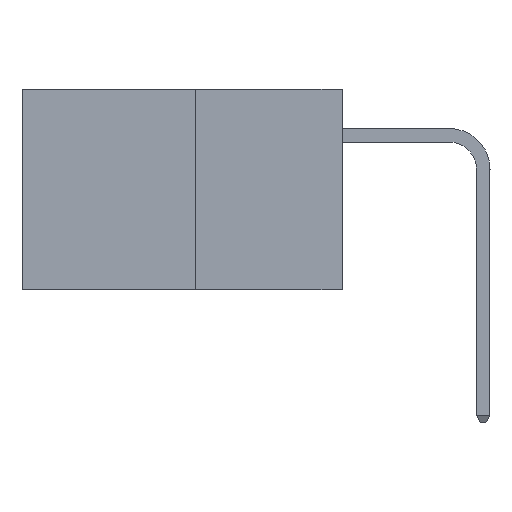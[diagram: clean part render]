
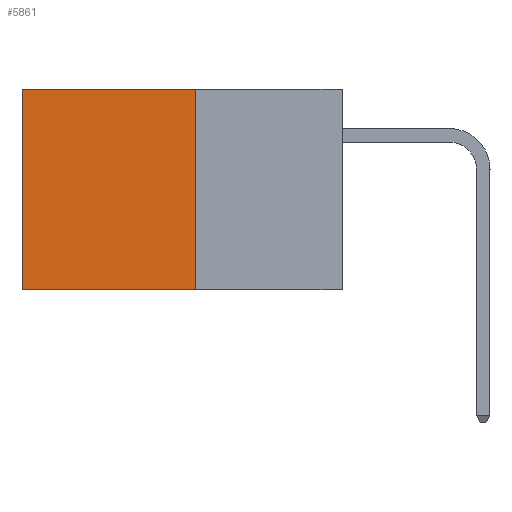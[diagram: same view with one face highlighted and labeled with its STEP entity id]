
A CAD part, left-side view. The second image highlights one B-rep face of the part: STEP entity #5861.
In plain terms, the highlighted planar face has unit normal (-1, 0, 0).
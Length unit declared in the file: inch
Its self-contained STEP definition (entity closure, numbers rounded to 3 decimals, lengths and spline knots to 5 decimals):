
#667 = VERTEX_POINT ( 'NONE', #10257 ) ;
#839 = CARTESIAN_POINT ( 'NONE',  ( 0.277, 0.27, 0. ) ) ;
#1763 = CARTESIAN_POINT ( 'NONE',  ( 0.277, 0.59, -0.37 ) ) ;
#1990 = CARTESIAN_POINT ( 'NONE',  ( 0.277, 0.59, 0. ) ) ;
#2166 = FACE_OUTER_BOUND ( 'NONE', #13178, .T. ) ;
#3160 = CARTESIAN_POINT ( 'NONE',  ( 0.277, 0.27, -0.37 ) ) ;
#3184 = VECTOR ( 'NONE', #15111, 39.37008 ) ;
#3936 = LINE ( 'NONE', #7426, #10573 ) ;
#4259 = LINE ( 'NONE', #15152, #3184 ) ;
#4852 = VERTEX_POINT ( 'NONE', #1763 ) ;
#4895 = DIRECTION ( 'NONE',  ( 0., 0., -1. ) ) ;
#4924 = ORIENTED_EDGE ( 'NONE', *, *, #10234, .T. ) ;
#5332 = AXIS2_PLACEMENT_3D ( 'NONE', #13194, #13041, #13023 ) ;
#5861 = ADVANCED_FACE ( 'NONE', ( #2166 ), #13466, .F. ) ;
#6286 = VECTOR ( 'NONE', #4895, 39.37008 ) ;
#6508 = EDGE_CURVE ( 'NONE', #667, #4852, #13981, .T. ) ;
#6579 = ORIENTED_EDGE ( 'NONE', *, *, #10232, .F. ) ;
#7426 = CARTESIAN_POINT ( 'NONE',  ( 0.277, 0.27, 0. ) ) ;
#7925 = ORIENTED_EDGE ( 'NONE', *, *, #8732, .T. ) ;
#8262 = ORIENTED_EDGE ( 'NONE', *, *, #6508, .F. ) ;
#8271 = VECTOR ( 'NONE', #12506, 39.37008 ) ;
#8302 = VERTEX_POINT ( 'NONE', #1990 ) ;
#8732 = EDGE_CURVE ( 'NONE', #11661, #8302, #3936, .T. ) ;
#9425 = LINE ( 'NONE', #10745, #6286 ) ;
#10232 = EDGE_CURVE ( 'NONE', #11661, #667, #4259, .T. ) ;
#10234 = EDGE_CURVE ( 'NONE', #8302, #4852, #9425, .T. ) ;
#10257 = CARTESIAN_POINT ( 'NONE',  ( 0.277, 0.27, -0.37 ) ) ;
#10573 = VECTOR ( 'NONE', #10827, 39.37008 ) ;
#10745 = CARTESIAN_POINT ( 'NONE',  ( 0.277, 0.59, -0.37 ) ) ;
#10827 = DIRECTION ( 'NONE',  ( 0., 1., 0. ) ) ;
#11661 = VERTEX_POINT ( 'NONE', #839 ) ;
#12506 = DIRECTION ( 'NONE',  ( 0., 1., 0. ) ) ;
#13023 = DIRECTION ( 'NONE',  ( 0., 0., -1. ) ) ;
#13041 = DIRECTION ( 'NONE',  ( 1., 0., 0. ) ) ;
#13178 = EDGE_LOOP ( 'NONE', ( #4924, #8262, #6579, #7925 ) ) ;
#13194 = CARTESIAN_POINT ( 'NONE',  ( 0.277, 0.27, -0.37 ) ) ;
#13466 = PLANE ( 'NONE',  #5332 ) ;
#13981 = LINE ( 'NONE', #3160, #8271 ) ;
#15111 = DIRECTION ( 'NONE',  ( 0., 0., -1. ) ) ;
#15152 = CARTESIAN_POINT ( 'NONE',  ( 0.277, 0.27, -0.37 ) ) ;
